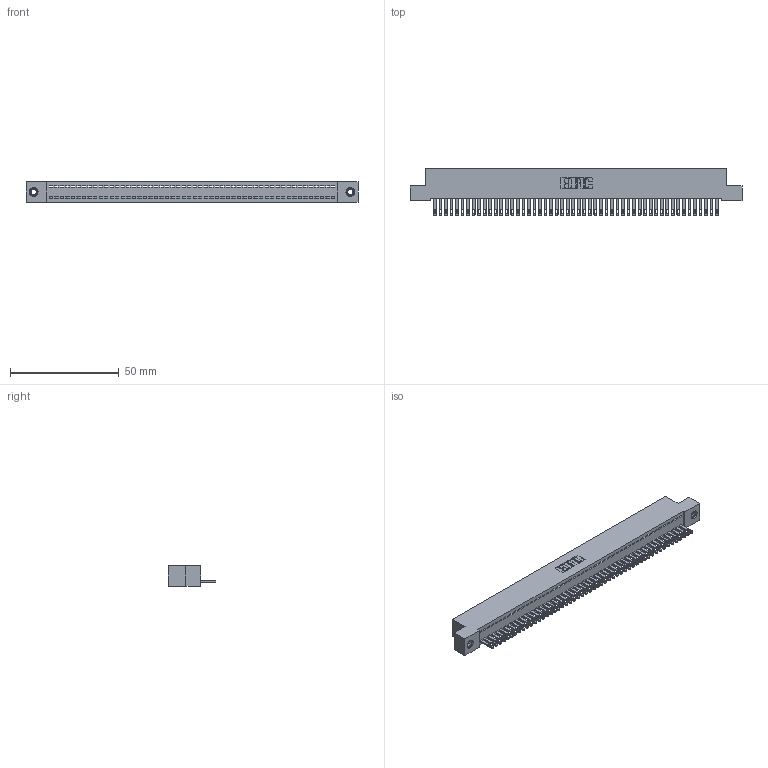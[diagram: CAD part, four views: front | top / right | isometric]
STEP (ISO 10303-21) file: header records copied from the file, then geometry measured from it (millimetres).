
FILE_DESCRIPTION (( 'STEP AP203' ), '1' );
FILE_NAME ('892-052-500-107.STEP', '2020-09-21T18:04:06', ( '' ), ( '' ), 'SwSTEP 2.0', 'SolidWorks 2020', '' );
FILE_SCHEMA (( 'CONFIG_CONTROL_DESIGN' ));
Length unit declared in the file: inch
Products named in the file (4): 345-250-001_345-250-005-103; 892-052-500-107; 842 Part_TI; 345-292-001_345-293-100
Assembly tree (55 placements, depth 2):
  892-052-500-107
    842 Part_TI
    345-292-001_345-293-100  x52
    345-250-001_345-250-005-103  x2
Bounding box: 152.4 x 21.85 x 9.4 mm (x, y, z)
Volume: 13418.8 mm3; surface area: 20026.1 mm2
Topology: 55 solids, 55 shells, 2978 faces, 9171 edges, 6106 vertices
Faces by surface type: plane 1970, cylinder 992, cone 12, torus 4
Entity records: 31480 total; most frequent: CARTESIAN_POINT 5409, ORIENTED_EDGE 5390, DIRECTION 4577, EDGE_CURVE 2695, LINE 2543, VECTOR 2543, VERTEX_POINT 1792, AXIS2_PLACEMENT_3D 1017
